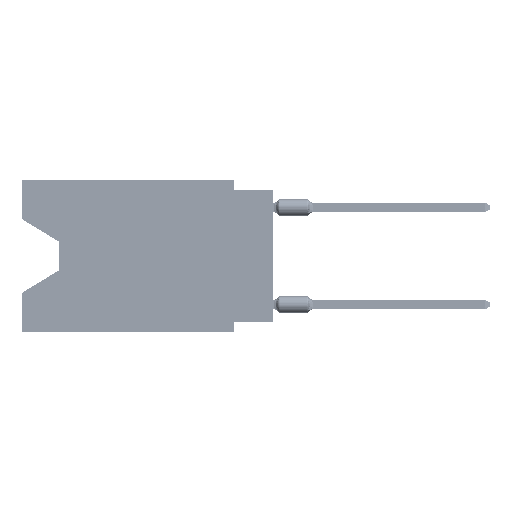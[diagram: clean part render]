
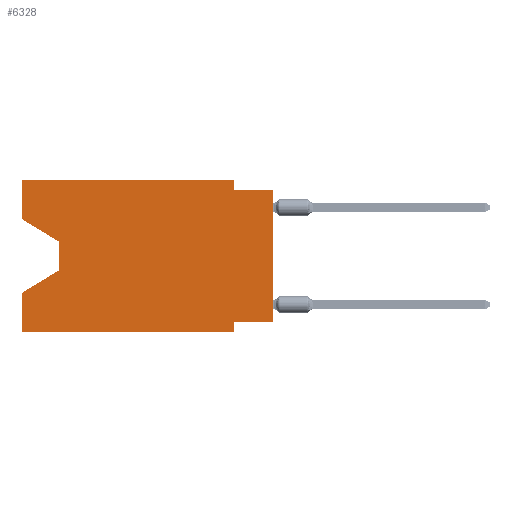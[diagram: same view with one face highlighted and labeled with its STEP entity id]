
A CAD part, left-side view. The second image highlights one B-rep face of the part: STEP entity #6328.
In plain terms, the highlighted planar face has unit normal (-1, 0, 0).
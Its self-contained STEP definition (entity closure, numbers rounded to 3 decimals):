
#70 = LINE ( 'NONE', #65847, #69351 ) ;
#615 = ORIENTED_EDGE ( 'NONE', *, *, #59055, .T. ) ;
#822 = CARTESIAN_POINT ( 'NONE',  ( 0., 2.54, 0. ) ) ;
#1359 = VECTOR ( 'NONE', #34565, 1000. ) ;
#2423 = CARTESIAN_POINT ( 'NONE',  ( 0., 16.383, -7.36 ) ) ;
#3301 = VECTOR ( 'NONE', #50139, 1000. ) ;
#3317 = EDGE_CURVE ( 'NONE', #21847, #35465, #7351, .T. ) ;
#3413 = VERTEX_POINT ( 'NONE', #63284 ) ;
#5472 = LINE ( 'NONE', #27668, #71774 ) ;
#6166 = EDGE_CURVE ( 'NONE', #14080, #18331, #24918, .T. ) ;
#6328 = ADVANCED_FACE ( 'NONE', ( #71748 ), #26709, .F. ) ;
#6980 = VECTOR ( 'NONE', #48753, 1000. ) ;
#7351 = LINE ( 'NONE', #822, #65912 ) ;
#8122 = VERTEX_POINT ( 'NONE', #17529 ) ;
#8206 = CARTESIAN_POINT ( 'NONE',  ( 0., 0., -0.635 ) ) ;
#8324 = CARTESIAN_POINT ( 'NONE',  ( 0., 16.383, 0. ) ) ;
#8472 = ORIENTED_EDGE ( 'NONE', *, *, #17109, .T. ) ;
#9832 = DIRECTION ( 'NONE',  ( 0., 0., 1. ) ) ;
#11084 = LINE ( 'NONE', #71786, #44947 ) ;
#13027 = CARTESIAN_POINT ( 'NONE',  ( 0., 13.97, -4.013 ) ) ;
#13068 = LINE ( 'NONE', #22563, #27889 ) ;
#13081 = EDGE_CURVE ( 'NONE', #24869, #8122, #11084, .T. ) ;
#13469 = ORIENTED_EDGE ( 'NONE', *, *, #3317, .F. ) ;
#14080 = VERTEX_POINT ( 'NONE', #36244 ) ;
#16149 = DIRECTION ( 'NONE',  ( 0., 0., -1. ) ) ;
#16705 = ORIENTED_EDGE ( 'NONE', *, *, #30673, .F. ) ;
#17109 = EDGE_CURVE ( 'NONE', #3413, #44844, #23316, .T. ) ;
#17360 = AXIS2_PLACEMENT_3D ( 'NONE', #21264, #65925, #16149 ) ;
#17529 = CARTESIAN_POINT ( 'NONE',  ( 0., 2.54, -9.906 ) ) ;
#18331 = VERTEX_POINT ( 'NONE', #23331 ) ;
#21264 = CARTESIAN_POINT ( 'NONE',  ( 0., 16.383, 0. ) ) ;
#21847 = VERTEX_POINT ( 'NONE', #61806 ) ;
#21966 = ORIENTED_EDGE ( 'NONE', *, *, #6166, .T. ) ;
#22172 = CARTESIAN_POINT ( 'NONE',  ( 0., 16.383, 0. ) ) ;
#22563 = CARTESIAN_POINT ( 'NONE',  ( 0., 0., -9.271 ) ) ;
#23316 = LINE ( 'NONE', #40368, #1359 ) ;
#23331 = CARTESIAN_POINT ( 'NONE',  ( 0., 0., -0.635 ) ) ;
#23854 = LINE ( 'NONE', #8206, #49604 ) ;
#24670 = DIRECTION ( 'NONE',  ( 0., 0., -1. ) ) ;
#24869 = VERTEX_POINT ( 'NONE', #28686 ) ;
#24918 = LINE ( 'NONE', #58690, #62581 ) ;
#26709 = PLANE ( 'NONE',  #17360 ) ;
#27668 = CARTESIAN_POINT ( 'NONE',  ( 0., 16.383, 0. ) ) ;
#27889 = VECTOR ( 'NONE', #62844, 1000. ) ;
#28487 = ORIENTED_EDGE ( 'NONE', *, *, #66047, .F. ) ;
#28625 = VERTEX_POINT ( 'NONE', #13027 ) ;
#28686 = CARTESIAN_POINT ( 'NONE',  ( 0., 16.383, -9.906 ) ) ;
#29528 = DIRECTION ( 'NONE',  ( 0., 0., -1. ) ) ;
#29888 = CARTESIAN_POINT ( 'NONE',  ( 0., 2.54, -0.635 ) ) ;
#30380 = DIRECTION ( 'NONE',  ( 0., -1., 0. ) ) ;
#30525 = ORIENTED_EDGE ( 'NONE', *, *, #58393, .F. ) ;
#30673 = EDGE_CURVE ( 'NONE', #63008, #8122, #65087, .T. ) ;
#32421 = EDGE_CURVE ( 'NONE', #24869, #44844, #57000, .T. ) ;
#34378 = VERTEX_POINT ( 'NONE', #8324 ) ;
#34565 = DIRECTION ( 'NONE',  ( 0., 0.855, -0.519 ) ) ;
#35219 = LINE ( 'NONE', #68620, #52085 ) ;
#35465 = VERTEX_POINT ( 'NONE', #29888 ) ;
#36244 = CARTESIAN_POINT ( 'NONE',  ( 0., 0., -9.271 ) ) ;
#38004 = DIRECTION ( 'NONE',  ( 0., -1., 0. ) ) ;
#40082 = ORIENTED_EDGE ( 'NONE', *, *, #45518, .F. ) ;
#40368 = CARTESIAN_POINT ( 'NONE',  ( 0., 13.97, -5.893 ) ) ;
#40412 = EDGE_LOOP ( 'NONE', ( #615, #67458, #8472, #54011, #49826, #16705, #40082, #21966, #30525, #13469, #43463, #28487 ) ) ;
#41330 = CARTESIAN_POINT ( 'NONE',  ( 0., 2.54, -9.271 ) ) ;
#41714 = CARTESIAN_POINT ( 'NONE',  ( 0., 16.383, -2.546 ) ) ;
#43463 = ORIENTED_EDGE ( 'NONE', *, *, #43813, .F. ) ;
#43813 = EDGE_CURVE ( 'NONE', #34378, #21847, #49774, .T. ) ;
#43983 = EDGE_CURVE ( 'NONE', #28625, #3413, #35219, .T. ) ;
#44844 = VERTEX_POINT ( 'NONE', #2423 ) ;
#44947 = VECTOR ( 'NONE', #38004, 1000. ) ;
#45518 = EDGE_CURVE ( 'NONE', #14080, #63008, #13068, .T. ) ;
#48753 = DIRECTION ( 'NONE',  ( 0., 0., -1. ) ) ;
#49604 = VECTOR ( 'NONE', #30380, 1000. ) ;
#49774 = LINE ( 'NONE', #22172, #3301 ) ;
#49826 = ORIENTED_EDGE ( 'NONE', *, *, #13081, .T. ) ;
#49875 = DIRECTION ( 'NONE',  ( 0., -0.855, -0.519 ) ) ;
#50139 = DIRECTION ( 'NONE',  ( 0., -1., 0. ) ) ;
#52085 = VECTOR ( 'NONE', #24670, 1000. ) ;
#54011 = ORIENTED_EDGE ( 'NONE', *, *, #32421, .F. ) ;
#56277 = CARTESIAN_POINT ( 'NONE',  ( 0., 16.383, 0. ) ) ;
#57000 = LINE ( 'NONE', #56277, #62831 ) ;
#58393 = EDGE_CURVE ( 'NONE', #35465, #18331, #23854, .T. ) ;
#58690 = CARTESIAN_POINT ( 'NONE',  ( 0., 0., 0. ) ) ;
#59055 = EDGE_CURVE ( 'NONE', #64178, #28625, #70, .T. ) ;
#59636 = CARTESIAN_POINT ( 'NONE',  ( 0., 2.54, -9.906 ) ) ;
#61374 = DIRECTION ( 'NONE',  ( 0., 0., 1. ) ) ;
#61806 = CARTESIAN_POINT ( 'NONE',  ( 0., 2.54, 0. ) ) ;
#62581 = VECTOR ( 'NONE', #70305, 1000. ) ;
#62831 = VECTOR ( 'NONE', #61374, 1000. ) ;
#62844 = DIRECTION ( 'NONE',  ( 0., 1., 0. ) ) ;
#63008 = VERTEX_POINT ( 'NONE', #41330 ) ;
#63284 = CARTESIAN_POINT ( 'NONE',  ( 0., 13.97, -5.893 ) ) ;
#64178 = VERTEX_POINT ( 'NONE', #41714 ) ;
#65087 = LINE ( 'NONE', #59636, #6980 ) ;
#65847 = CARTESIAN_POINT ( 'NONE',  ( 0., 16.383, -2.546 ) ) ;
#65912 = VECTOR ( 'NONE', #29528, 1000. ) ;
#65925 = DIRECTION ( 'NONE',  ( 1., 0., 0. ) ) ;
#66047 = EDGE_CURVE ( 'NONE', #64178, #34378, #5472, .T. ) ;
#67458 = ORIENTED_EDGE ( 'NONE', *, *, #43983, .T. ) ;
#68620 = CARTESIAN_POINT ( 'NONE',  ( 0., 13.97, -4.013 ) ) ;
#69351 = VECTOR ( 'NONE', #49875, 1000. ) ;
#70305 = DIRECTION ( 'NONE',  ( 0., 0., 1. ) ) ;
#71748 = FACE_OUTER_BOUND ( 'NONE', #40412, .T. ) ;
#71774 = VECTOR ( 'NONE', #9832, 1000. ) ;
#71786 = CARTESIAN_POINT ( 'NONE',  ( 0., 16.383, -9.906 ) ) ;
